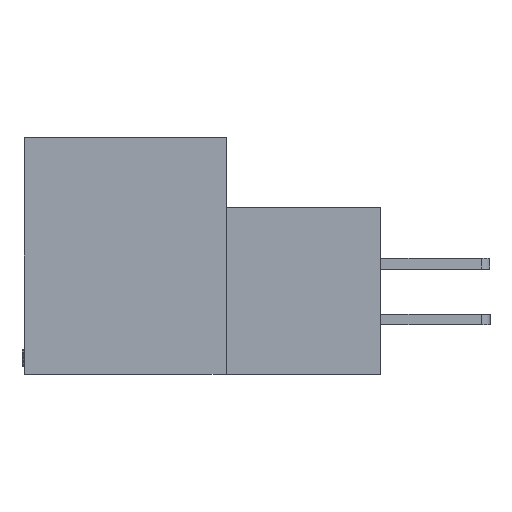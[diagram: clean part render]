
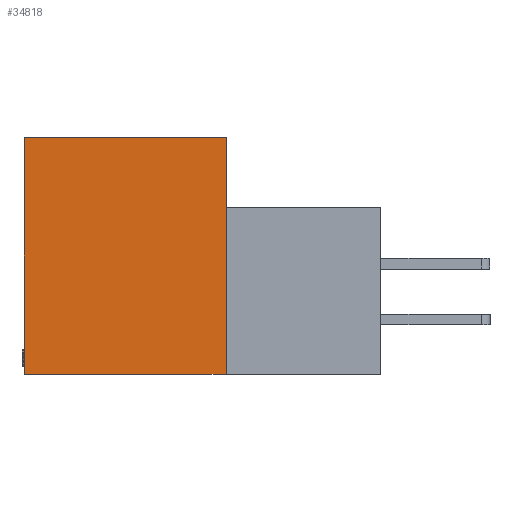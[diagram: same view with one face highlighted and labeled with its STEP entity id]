
A CAD part, left-side view. The second image highlights one B-rep face of the part: STEP entity #34818.
In plain terms, the highlighted planar face has unit normal (-1, 0, 0).
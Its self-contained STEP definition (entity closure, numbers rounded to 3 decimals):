
#4112 = CARTESIAN_POINT ( 'NONE',  ( 0., 11.506, 0. ) ) ;
#4749 = DIRECTION ( 'NONE',  ( 1., 0., 0. ) ) ;
#5012 = VERTEX_POINT ( 'NONE', #37562 ) ;
#5180 = CARTESIAN_POINT ( 'NONE',  ( 0., 0., 0. ) ) ;
#5551 = VERTEX_POINT ( 'NONE', #39356 ) ;
#7405 = VECTOR ( 'NONE', #13953, 1000. ) ;
#7500 = EDGE_CURVE ( 'NONE', #5012, #5551, #13015, .T. ) ;
#7933 = CARTESIAN_POINT ( 'NONE',  ( 0., 11.506, 0. ) ) ;
#8248 = VECTOR ( 'NONE', #18741, 1000. ) ;
#10784 = EDGE_CURVE ( 'NONE', #5551, #15602, #35138, .T. ) ;
#11438 = PLANE ( 'NONE',  #18881 ) ;
#12464 = CARTESIAN_POINT ( 'NONE',  ( 0., 0., 0. ) ) ;
#13015 = LINE ( 'NONE', #25537, #17924 ) ;
#13921 = ORIENTED_EDGE ( 'NONE', *, *, #15620, .F. ) ;
#13953 = DIRECTION ( 'NONE',  ( 0., -1., 0. ) ) ;
#14307 = DIRECTION ( 'NONE',  ( 0., 0., -1. ) ) ;
#15602 = VERTEX_POINT ( 'NONE', #4112 ) ;
#15620 = EDGE_CURVE ( 'NONE', #15602, #28872, #37625, .T. ) ;
#16388 = DIRECTION ( 'NONE',  ( 0., 0., 1. ) ) ;
#17179 = ORIENTED_EDGE ( 'NONE', *, *, #7500, .F. ) ;
#17413 = EDGE_CURVE ( 'NONE', #28872, #5012, #22405, .T. ) ;
#17924 = VECTOR ( 'NONE', #31940, 1000. ) ;
#18741 = DIRECTION ( 'NONE',  ( 0., 0., -1. ) ) ;
#18881 = AXIS2_PLACEMENT_3D ( 'NONE', #5180, #4749, #14307 ) ;
#18924 = EDGE_LOOP ( 'NONE', ( #17179, #39541, #13921, #23653 ) ) ;
#20593 = FACE_OUTER_BOUND ( 'NONE', #18924, .T. ) ;
#22405 = LINE ( 'NONE', #12464, #8248 ) ;
#23653 = ORIENTED_EDGE ( 'NONE', *, *, #10784, .F. ) ;
#25537 = CARTESIAN_POINT ( 'NONE',  ( 0., -8.814, -13.487 ) ) ;
#26851 = VECTOR ( 'NONE', #16388, 1000. ) ;
#28872 = VERTEX_POINT ( 'NONE', #39844 ) ;
#29164 = CARTESIAN_POINT ( 'NONE',  ( 0., 11.506, -13.487 ) ) ;
#31940 = DIRECTION ( 'NONE',  ( 0., 1., 0. ) ) ;
#34818 = ADVANCED_FACE ( 'NONE', ( #20593 ), #11438, .F. ) ;
#35138 = LINE ( 'NONE', #29164, #26851 ) ;
#37562 = CARTESIAN_POINT ( 'NONE',  ( 0., 0., -13.487 ) ) ;
#37625 = LINE ( 'NONE', #7933, #7405 ) ;
#39356 = CARTESIAN_POINT ( 'NONE',  ( 0., 11.506, -13.487 ) ) ;
#39541 = ORIENTED_EDGE ( 'NONE', *, *, #17413, .F. ) ;
#39844 = CARTESIAN_POINT ( 'NONE',  ( 0., 0., 0. ) ) ;
